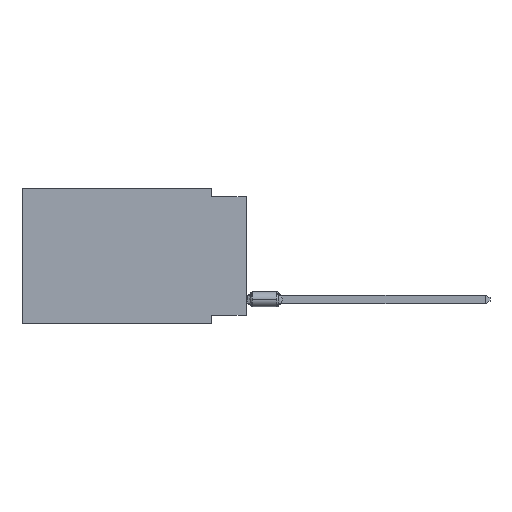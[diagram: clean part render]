
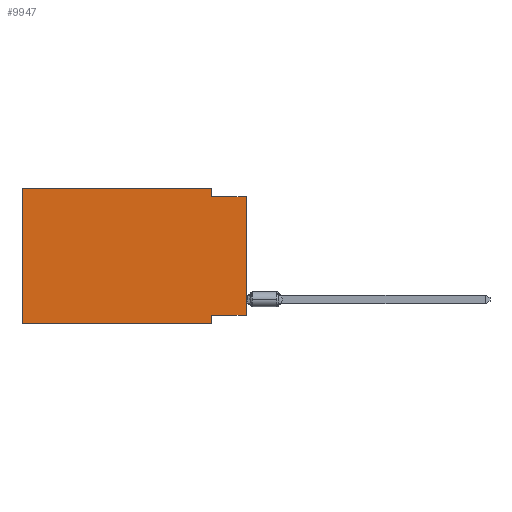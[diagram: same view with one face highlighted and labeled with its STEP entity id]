
A CAD part, left-side view. The second image highlights one B-rep face of the part: STEP entity #9947.
In plain terms, the highlighted planar face has unit normal (-1, 0, 0).
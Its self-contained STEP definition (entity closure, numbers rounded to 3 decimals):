
#125 = EDGE_LOOP ( 'NONE', ( #1352, #11377, #8964, #16585, #15340, #17166, #15749, #17649 ) ) ;
#288 = VECTOR ( 'NONE', #6834, 1000. ) ;
#445 = CARTESIAN_POINT ( 'NONE',  ( 0., 2.54, -9.906 ) ) ;
#1352 = ORIENTED_EDGE ( 'NONE', *, *, #1841, .T. ) ;
#1821 = CARTESIAN_POINT ( 'NONE',  ( 0., 0., -0.635 ) ) ;
#1841 = EDGE_CURVE ( 'NONE', #14954, #14580, #15288, .T. ) ;
#2188 = AXIS2_PLACEMENT_3D ( 'NONE', #9507, #15144, #2478 ) ;
#2478 = DIRECTION ( 'NONE',  ( 0., 0., -1. ) ) ;
#2564 = VECTOR ( 'NONE', #3436, 1000. ) ;
#3176 = EDGE_CURVE ( 'NONE', #16266, #13329, #8827, .T. ) ;
#3426 = CARTESIAN_POINT ( 'NONE',  ( 0., 0., -0.635 ) ) ;
#3436 = DIRECTION ( 'NONE',  ( 0., 0., -1. ) ) ;
#3785 = CARTESIAN_POINT ( 'NONE',  ( 0., 0., -9.271 ) ) ;
#4107 = VECTOR ( 'NONE', #17083, 1000. ) ;
#4164 = CARTESIAN_POINT ( 'NONE',  ( 0., 16.383, -9.906 ) ) ;
#4499 = CARTESIAN_POINT ( 'NONE',  ( 0., 16.383, 0. ) ) ;
#4571 = DIRECTION ( 'NONE',  ( 0., -1., 0. ) ) ;
#5219 = EDGE_CURVE ( 'NONE', #15768, #16266, #15394, .T. ) ;
#5776 = CARTESIAN_POINT ( 'NONE',  ( 0., 2.54, -9.906 ) ) ;
#5914 = VECTOR ( 'NONE', #13915, 1000. ) ;
#6489 = EDGE_CURVE ( 'NONE', #13698, #11470, #11811, .T. ) ;
#6834 = DIRECTION ( 'NONE',  ( 0., 1., 0. ) ) ;
#6965 = DIRECTION ( 'NONE',  ( 0., 0., 1. ) ) ;
#7113 = CARTESIAN_POINT ( 'NONE',  ( 0., 16.383, -9.906 ) ) ;
#7405 = CARTESIAN_POINT ( 'NONE',  ( 0., 2.54, 0. ) ) ;
#7652 = CARTESIAN_POINT ( 'NONE',  ( 0., 0., -9.271 ) ) ;
#7991 = CARTESIAN_POINT ( 'NONE',  ( 0., 0., 0. ) ) ;
#8372 = CARTESIAN_POINT ( 'NONE',  ( 0., 16.383, 0. ) ) ;
#8740 = LINE ( 'NONE', #1821, #15748 ) ;
#8827 = LINE ( 'NONE', #11711, #4107 ) ;
#8964 = ORIENTED_EDGE ( 'NONE', *, *, #17204, .F. ) ;
#8996 = LINE ( 'NONE', #10570, #2564 ) ;
#9071 = PLANE ( 'NONE',  #2188 ) ;
#9507 = CARTESIAN_POINT ( 'NONE',  ( 0., 16.383, 0. ) ) ;
#9947 = ADVANCED_FACE ( 'NONE', ( #14706 ), #9071, .F. ) ;
#10211 = VERTEX_POINT ( 'NONE', #15876 ) ;
#10240 = DIRECTION ( 'NONE',  ( 0., 0., -1. ) ) ;
#10570 = CARTESIAN_POINT ( 'NONE',  ( 0., 2.54, 0. ) ) ;
#11016 = LINE ( 'NONE', #3785, #288 ) ;
#11377 = ORIENTED_EDGE ( 'NONE', *, *, #11692, .F. ) ;
#11470 = VERTEX_POINT ( 'NONE', #5776 ) ;
#11692 = EDGE_CURVE ( 'NONE', #10211, #14580, #8740, .T. ) ;
#11711 = CARTESIAN_POINT ( 'NONE',  ( 0., 16.383, 0. ) ) ;
#11811 = LINE ( 'NONE', #445, #16842 ) ;
#13329 = VERTEX_POINT ( 'NONE', #7405 ) ;
#13401 = EDGE_CURVE ( 'NONE', #14954, #13698, #11016, .T. ) ;
#13638 = LINE ( 'NONE', #7113, #13990 ) ;
#13698 = VERTEX_POINT ( 'NONE', #14770 ) ;
#13884 = VECTOR ( 'NONE', #6965, 1000. ) ;
#13915 = DIRECTION ( 'NONE',  ( 0., 0., 1. ) ) ;
#13990 = VECTOR ( 'NONE', #17894, 1000. ) ;
#14580 = VERTEX_POINT ( 'NONE', #3426 ) ;
#14706 = FACE_OUTER_BOUND ( 'NONE', #125, .T. ) ;
#14770 = CARTESIAN_POINT ( 'NONE',  ( 0., 2.54, -9.271 ) ) ;
#14954 = VERTEX_POINT ( 'NONE', #7652 ) ;
#15144 = DIRECTION ( 'NONE',  ( 1., 0., 0. ) ) ;
#15288 = LINE ( 'NONE', #7991, #5914 ) ;
#15340 = ORIENTED_EDGE ( 'NONE', *, *, #5219, .F. ) ;
#15394 = LINE ( 'NONE', #8372, #13884 ) ;
#15706 = EDGE_CURVE ( 'NONE', #15768, #11470, #13638, .T. ) ;
#15748 = VECTOR ( 'NONE', #4571, 1000. ) ;
#15749 = ORIENTED_EDGE ( 'NONE', *, *, #6489, .F. ) ;
#15768 = VERTEX_POINT ( 'NONE', #4164 ) ;
#15876 = CARTESIAN_POINT ( 'NONE',  ( 0., 2.54, -0.635 ) ) ;
#16266 = VERTEX_POINT ( 'NONE', #4499 ) ;
#16585 = ORIENTED_EDGE ( 'NONE', *, *, #3176, .F. ) ;
#16842 = VECTOR ( 'NONE', #10240, 1000. ) ;
#17083 = DIRECTION ( 'NONE',  ( 0., -1., 0. ) ) ;
#17166 = ORIENTED_EDGE ( 'NONE', *, *, #15706, .T. ) ;
#17204 = EDGE_CURVE ( 'NONE', #13329, #10211, #8996, .T. ) ;
#17649 = ORIENTED_EDGE ( 'NONE', *, *, #13401, .F. ) ;
#17894 = DIRECTION ( 'NONE',  ( 0., -1., 0. ) ) ;
